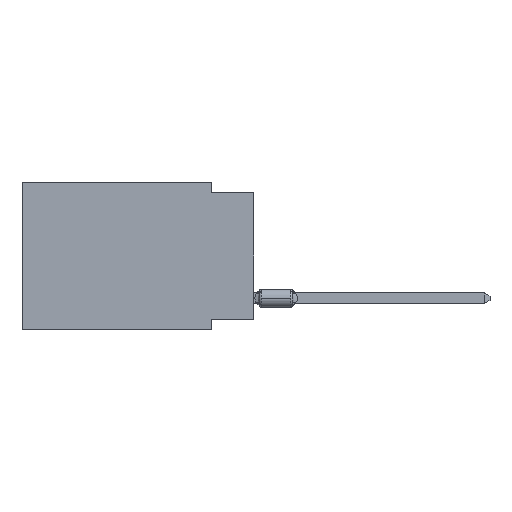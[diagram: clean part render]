
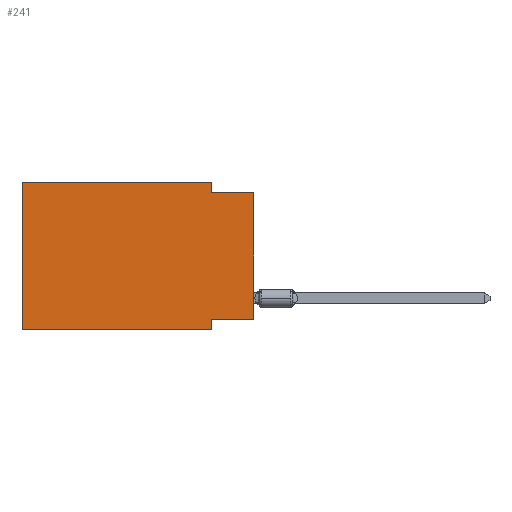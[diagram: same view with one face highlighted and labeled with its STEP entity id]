
A CAD part, left-side view. The second image highlights one B-rep face of the part: STEP entity #241.
In plain terms, the highlighted planar face has unit normal (-1, 0, 0).
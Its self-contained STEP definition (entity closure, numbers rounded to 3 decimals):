
#128 = EDGE_CURVE ( 'NONE', #4940, #6037, #4278, .T. ) ;
#241 = ADVANCED_FACE ( 'NONE', ( #20853 ), #6163, .F. ) ;
#889 = CARTESIAN_POINT ( 'NONE',  ( 0., 2.54, 0. ) ) ;
#948 = VERTEX_POINT ( 'NONE', #14714 ) ;
#1368 = LINE ( 'NONE', #4670, #21155 ) ;
#1430 = ORIENTED_EDGE ( 'NONE', *, *, #128, .T. ) ;
#1983 = LINE ( 'NONE', #19984, #3839 ) ;
#2226 = DIRECTION ( 'NONE',  ( 0., -1., 0. ) ) ;
#2265 = VECTOR ( 'NONE', #10269, 1000. ) ;
#2280 = EDGE_LOOP ( 'NONE', ( #19490, #19301, #17505, #16439, #11174, #1430, #17668, #3034 ) ) ;
#3034 = ORIENTED_EDGE ( 'NONE', *, *, #19978, .F. ) ;
#3153 = CARTESIAN_POINT ( 'NONE',  ( 0., 13.97, -8.89 ) ) ;
#3378 = DIRECTION ( 'NONE',  ( 0., -1., 0. ) ) ;
#3458 = CARTESIAN_POINT ( 'NONE',  ( 0., 0., 0. ) ) ;
#3711 = CARTESIAN_POINT ( 'NONE',  ( 0., 13.97, 0. ) ) ;
#3839 = VECTOR ( 'NONE', #11500, 1000. ) ;
#4278 = LINE ( 'NONE', #17127, #20446 ) ;
#4670 = CARTESIAN_POINT ( 'NONE',  ( 0., 0., -0.635 ) ) ;
#4839 = VERTEX_POINT ( 'NONE', #6517 ) ;
#4940 = VERTEX_POINT ( 'NONE', #3153 ) ;
#5192 = DIRECTION ( 'NONE',  ( 0., 0., 1. ) ) ;
#5877 = CARTESIAN_POINT ( 'NONE',  ( 0., 2.54, -8.89 ) ) ;
#5978 = LINE ( 'NONE', #17047, #11135 ) ;
#6037 = VERTEX_POINT ( 'NONE', #5877 ) ;
#6163 = PLANE ( 'NONE',  #19088 ) ;
#6517 = CARTESIAN_POINT ( 'NONE',  ( 0., 0., -0.635 ) ) ;
#7066 = EDGE_CURVE ( 'NONE', #9138, #6037, #5978, .T. ) ;
#7193 = VERTEX_POINT ( 'NONE', #9290 ) ;
#7485 = VECTOR ( 'NONE', #3378, 1000. ) ;
#8444 = CARTESIAN_POINT ( 'NONE',  ( 0., 2.54, -8.255 ) ) ;
#9138 = VERTEX_POINT ( 'NONE', #8444 ) ;
#9290 = CARTESIAN_POINT ( 'NONE',  ( 0., 0., -8.255 ) ) ;
#9846 = EDGE_CURVE ( 'NONE', #4940, #10012, #11408, .T. ) ;
#10012 = VERTEX_POINT ( 'NONE', #3711 ) ;
#10269 = DIRECTION ( 'NONE',  ( 0., 0., 1. ) ) ;
#11135 = VECTOR ( 'NONE', #20453, 1000. ) ;
#11174 = ORIENTED_EDGE ( 'NONE', *, *, #9846, .F. ) ;
#11408 = LINE ( 'NONE', #14641, #14694 ) ;
#11500 = DIRECTION ( 'NONE',  ( 0., 0., -1. ) ) ;
#11562 = EDGE_CURVE ( 'NONE', #17384, #948, #1983, .T. ) ;
#13206 = CARTESIAN_POINT ( 'NONE',  ( 0., 13.97, 0. ) ) ;
#14641 = CARTESIAN_POINT ( 'NONE',  ( 0., 13.97, 0. ) ) ;
#14694 = VECTOR ( 'NONE', #5192, 1000. ) ;
#14714 = CARTESIAN_POINT ( 'NONE',  ( 0., 2.54, -0.635 ) ) ;
#16430 = LINE ( 'NONE', #3458, #2265 ) ;
#16439 = ORIENTED_EDGE ( 'NONE', *, *, #18812, .F. ) ;
#17047 = CARTESIAN_POINT ( 'NONE',  ( 0., 2.54, -8.89 ) ) ;
#17127 = CARTESIAN_POINT ( 'NONE',  ( 0., 13.97, -8.89 ) ) ;
#17384 = VERTEX_POINT ( 'NONE', #889 ) ;
#17505 = ORIENTED_EDGE ( 'NONE', *, *, #11562, .F. ) ;
#17657 = CARTESIAN_POINT ( 'NONE',  ( 0., 0., -8.255 ) ) ;
#17661 = DIRECTION ( 'NONE',  ( 0., 0., -1. ) ) ;
#17668 = ORIENTED_EDGE ( 'NONE', *, *, #7066, .F. ) ;
#17863 = DIRECTION ( 'NONE',  ( 0., 1., 0. ) ) ;
#18737 = EDGE_CURVE ( 'NONE', #948, #4839, #1368, .T. ) ;
#18812 = EDGE_CURVE ( 'NONE', #10012, #17384, #19550, .T. ) ;
#19088 = AXIS2_PLACEMENT_3D ( 'NONE', #20956, #19253, #17661 ) ;
#19206 = EDGE_CURVE ( 'NONE', #7193, #4839, #16430, .T. ) ;
#19247 = LINE ( 'NONE', #17657, #19728 ) ;
#19253 = DIRECTION ( 'NONE',  ( 1., 0., 0. ) ) ;
#19301 = ORIENTED_EDGE ( 'NONE', *, *, #18737, .F. ) ;
#19490 = ORIENTED_EDGE ( 'NONE', *, *, #19206, .T. ) ;
#19550 = LINE ( 'NONE', #13206, #7485 ) ;
#19728 = VECTOR ( 'NONE', #17863, 1000. ) ;
#19978 = EDGE_CURVE ( 'NONE', #7193, #9138, #19247, .T. ) ;
#19984 = CARTESIAN_POINT ( 'NONE',  ( 0., 2.54, 0. ) ) ;
#20446 = VECTOR ( 'NONE', #2226, 1000. ) ;
#20453 = DIRECTION ( 'NONE',  ( 0., 0., -1. ) ) ;
#20853 = FACE_OUTER_BOUND ( 'NONE', #2280, .T. ) ;
#20956 = CARTESIAN_POINT ( 'NONE',  ( 0., 13.97, 0. ) ) ;
#21152 = DIRECTION ( 'NONE',  ( 0., -1., 0. ) ) ;
#21155 = VECTOR ( 'NONE', #21152, 1000. ) ;
